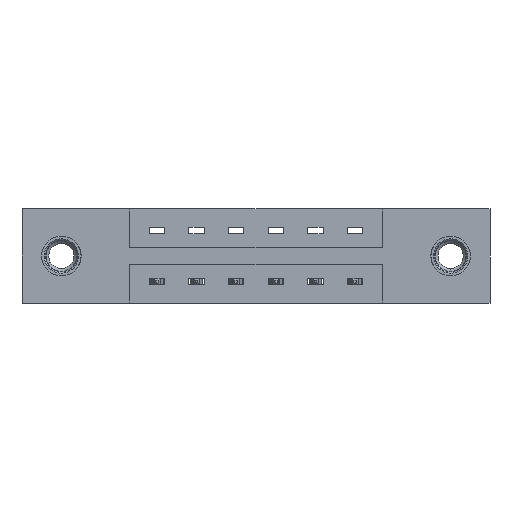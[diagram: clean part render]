
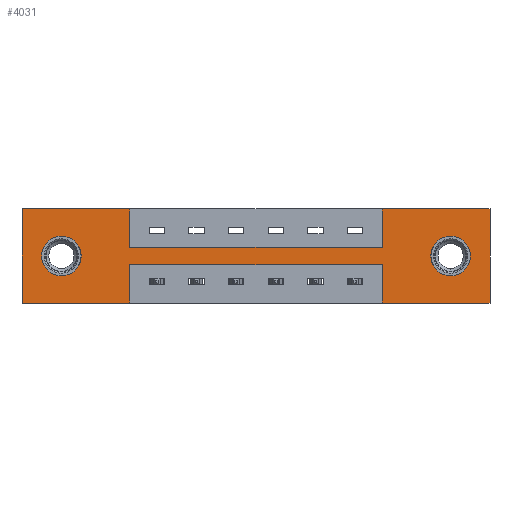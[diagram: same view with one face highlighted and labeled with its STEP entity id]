
A CAD part, front view. The second image highlights one B-rep face of the part: STEP entity #4031.
In plain terms, the highlighted planar face has unit normal (0, -1, 0).
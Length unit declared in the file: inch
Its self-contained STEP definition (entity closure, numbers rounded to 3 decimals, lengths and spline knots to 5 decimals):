
#107 = VECTOR ( 'NONE', #5665, 39.37008 ) ;
#125 = CARTESIAN_POINT ( 'NONE',  ( 0.425, 0., 0. ) ) ;
#155 = CARTESIAN_POINT ( 'NONE',  ( 1.842, 0., 0. ) ) ;
#157 = VERTEX_POINT ( 'NONE', #7164 ) ;
#264 = LINE ( 'NONE', #3424, #6249 ) ;
#421 = FACE_OUTER_BOUND ( 'NONE', #9651, .T. ) ;
#451 = DIRECTION ( 'NONE',  ( 0., 0., 1. ) ) ;
#482 = VERTEX_POINT ( 'NONE', #5175 ) ;
#483 = ORIENTED_EDGE ( 'NONE', *, *, #7003, .T. ) ;
#486 = LINE ( 'NONE', #1958, #2601 ) ;
#682 = VECTOR ( 'NONE', #8578, 39.37008 ) ;
#704 = LINE ( 'NONE', #2115, #1586 ) ;
#732 = DIRECTION ( 'NONE',  ( 0., 0., -1. ) ) ;
#839 = LINE ( 'NONE', #4768, #1840 ) ;
#875 = EDGE_CURVE ( 'NONE', #3739, #8464, #264, .T. ) ;
#1070 = VECTOR ( 'NONE', #9857, 39.37008 ) ;
#1173 = ORIENTED_EDGE ( 'NONE', *, *, #875, .F. ) ;
#1215 = VERTEX_POINT ( 'NONE', #9106 ) ;
#1236 = AXIS2_PLACEMENT_3D ( 'NONE', #1918, #8223, #9912 ) ;
#1338 = CARTESIAN_POINT ( 'NONE',  ( 0.425, 0., -0.37 ) ) ;
#1411 = EDGE_LOOP ( 'NONE', ( #483, #3594 ) ) ;
#1547 = EDGE_CURVE ( 'NONE', #9848, #2451, #4729, .T. ) ;
#1586 = VECTOR ( 'NONE', #451, 39.37008 ) ;
#1597 = DIRECTION ( 'NONE',  ( 0., 0., 1. ) ) ;
#1738 = VERTEX_POINT ( 'NONE', #2378 ) ;
#1745 = VERTEX_POINT ( 'NONE', #4076 ) ;
#1784 = DIRECTION ( 'NONE',  ( 0., 0., 1. ) ) ;
#1840 = VECTOR ( 'NONE', #1597, 39.37008 ) ;
#1918 = CARTESIAN_POINT ( 'NONE',  ( 1.687, 0., -0.185 ) ) ;
#1941 = DIRECTION ( 'NONE',  ( 0., -1., 0. ) ) ;
#1958 = CARTESIAN_POINT ( 'NONE',  ( 0., 0., -0.37 ) ) ;
#2009 = CARTESIAN_POINT ( 'NONE',  ( 0., 0., -0.37 ) ) ;
#2115 = CARTESIAN_POINT ( 'NONE',  ( 1.417, 0., 0. ) ) ;
#2192 = EDGE_CURVE ( 'NONE', #8464, #482, #3199, .T. ) ;
#2226 = DIRECTION ( 'NONE',  ( 1., 0., 0. ) ) ;
#2378 = CARTESIAN_POINT ( 'NONE',  ( 1.417, 0., -0.37 ) ) ;
#2384 = ORIENTED_EDGE ( 'NONE', *, *, #6631, .F. ) ;
#2394 = DIRECTION ( 'NONE',  ( 0., 1., 0. ) ) ;
#2451 = VERTEX_POINT ( 'NONE', #5269 ) ;
#2475 = EDGE_CURVE ( 'NONE', #482, #9816, #704, .T. ) ;
#2498 = CARTESIAN_POINT ( 'NONE',  ( 0.425, 0., -0.22 ) ) ;
#2515 = ORIENTED_EDGE ( 'NONE', *, *, #2475, .F. ) ;
#2528 = FACE_BOUND ( 'NONE', #1411, .T. ) ;
#2574 = CARTESIAN_POINT ( 'NONE',  ( 0., 0., 0. ) ) ;
#2601 = VECTOR ( 'NONE', #7566, 39.37008 ) ;
#2655 = CIRCLE ( 'NONE', #9099, 0.078 ) ;
#2710 = CIRCLE ( 'NONE', #3283, 0.078 ) ;
#2769 = LINE ( 'NONE', #2574, #5396 ) ;
#2834 = LINE ( 'NONE', #3782, #3086 ) ;
#2854 = LINE ( 'NONE', #5039, #9895 ) ;
#3024 = FACE_BOUND ( 'NONE', #3153, .T. ) ;
#3029 = CARTESIAN_POINT ( 'NONE',  ( 0.425, 0., -0.15 ) ) ;
#3086 = VECTOR ( 'NONE', #2226, 39.37008 ) ;
#3153 = EDGE_LOOP ( 'NONE', ( #8442, #5139 ) ) ;
#3199 = LINE ( 'NONE', #4795, #107 ) ;
#3210 = EDGE_CURVE ( 'NONE', #7838, #157, #9429, .T. ) ;
#3283 = AXIS2_PLACEMENT_3D ( 'NONE', #8961, #9764, #1784 ) ;
#3424 = CARTESIAN_POINT ( 'NONE',  ( 0.425, 0., 0. ) ) ;
#3465 = DIRECTION ( 'NONE',  ( 0., 0., -1. ) ) ;
#3594 = ORIENTED_EDGE ( 'NONE', *, *, #3713, .T. ) ;
#3713 = EDGE_CURVE ( 'NONE', #6350, #4746, #2655, .T. ) ;
#3739 = VERTEX_POINT ( 'NONE', #125 ) ;
#3782 = CARTESIAN_POINT ( 'NONE',  ( 0., 0., 0. ) ) ;
#3869 = VECTOR ( 'NONE', #6880, 39.37008 ) ;
#4019 = VECTOR ( 'NONE', #7086, 39.37008 ) ;
#4031 = ADVANCED_FACE ( 'NONE', ( #3024, #2528, #421 ), #8391, .T. ) ;
#4065 = DIRECTION ( 'NONE',  ( 1., 0., 0. ) ) ;
#4076 = CARTESIAN_POINT ( 'NONE',  ( 1.417, 0., -0.22 ) ) ;
#4135 = ORIENTED_EDGE ( 'NONE', *, *, #6311, .F. ) ;
#4234 = DIRECTION ( 'NONE',  ( 0., 0., -1. ) ) ;
#4255 = EDGE_CURVE ( 'NONE', #2451, #9848, #7679, .T. ) ;
#4355 = EDGE_CURVE ( 'NONE', #9816, #7743, #2769, .T. ) ;
#4473 = VERTEX_POINT ( 'NONE', #7274 ) ;
#4729 = CIRCLE ( 'NONE', #1236, 0.078 ) ;
#4732 = CARTESIAN_POINT ( 'NONE',  ( 0., 0., 0. ) ) ;
#4739 = AXIS2_PLACEMENT_3D ( 'NONE', #9506, #2394, #732 ) ;
#4746 = VERTEX_POINT ( 'NONE', #6963 ) ;
#4768 = CARTESIAN_POINT ( 'NONE',  ( 1.417, 0., -0.37 ) ) ;
#4795 = CARTESIAN_POINT ( 'NONE',  ( 0.425, 0., -0.15 ) ) ;
#4933 = CARTESIAN_POINT ( 'NONE',  ( 1.687, 0., -0.263 ) ) ;
#5039 = CARTESIAN_POINT ( 'NONE',  ( 1.842, 0., 0. ) ) ;
#5139 = ORIENTED_EDGE ( 'NONE', *, *, #1547, .T. ) ;
#5154 = EDGE_CURVE ( 'NONE', #4473, #1738, #8388, .T. ) ;
#5175 = CARTESIAN_POINT ( 'NONE',  ( 1.417, 0., -0.15 ) ) ;
#5269 = CARTESIAN_POINT ( 'NONE',  ( 1.687, 0., -0.107 ) ) ;
#5276 = CARTESIAN_POINT ( 'NONE',  ( 0., 0., -0.37 ) ) ;
#5392 = ORIENTED_EDGE ( 'NONE', *, *, #5154, .F. ) ;
#5396 = VECTOR ( 'NONE', #4065, 39.37008 ) ;
#5573 = DIRECTION ( 'NONE',  ( 0., 0., 1. ) ) ;
#5665 = DIRECTION ( 'NONE',  ( 1., 0., 0. ) ) ;
#5760 = CARTESIAN_POINT ( 'NONE',  ( 1.417, 0., 0. ) ) ;
#6031 = EDGE_CURVE ( 'NONE', #8325, #1215, #8273, .T. ) ;
#6127 = CARTESIAN_POINT ( 'NONE',  ( 0., 0., -0.37 ) ) ;
#6249 = VECTOR ( 'NONE', #4234, 39.37008 ) ;
#6311 = EDGE_CURVE ( 'NONE', #7743, #4473, #2854, .T. ) ;
#6350 = VERTEX_POINT ( 'NONE', #6685 ) ;
#6411 = DIRECTION ( 'NONE',  ( 0., 1., 0. ) ) ;
#6590 = LINE ( 'NONE', #7442, #1070 ) ;
#6631 = EDGE_CURVE ( 'NONE', #157, #8325, #486, .T. ) ;
#6685 = CARTESIAN_POINT ( 'NONE',  ( 0.155, 0., -0.263 ) ) ;
#6880 = DIRECTION ( 'NONE',  ( -1., 0., 0. ) ) ;
#6963 = CARTESIAN_POINT ( 'NONE',  ( 0.155, 0., -0.107 ) ) ;
#7003 = EDGE_CURVE ( 'NONE', #4746, #6350, #2710, .T. ) ;
#7062 = ORIENTED_EDGE ( 'NONE', *, *, #3210, .F. ) ;
#7086 = DIRECTION ( 'NONE',  ( 0., 0., 1. ) ) ;
#7164 = CARTESIAN_POINT ( 'NONE',  ( 0.425, 0., -0.37 ) ) ;
#7246 = ORIENTED_EDGE ( 'NONE', *, *, #4355, .F. ) ;
#7274 = CARTESIAN_POINT ( 'NONE',  ( 1.842, 0., -0.37 ) ) ;
#7296 = AXIS2_PLACEMENT_3D ( 'NONE', #2009, #1941, #8351 ) ;
#7442 = CARTESIAN_POINT ( 'NONE',  ( 0.425, 0., -0.22 ) ) ;
#7566 = DIRECTION ( 'NONE',  ( -1., 0., 0. ) ) ;
#7661 = EDGE_CURVE ( 'NONE', #1215, #3739, #2834, .T. ) ;
#7679 = CIRCLE ( 'NONE', #4739, 0.078 ) ;
#7743 = VERTEX_POINT ( 'NONE', #155 ) ;
#7826 = ORIENTED_EDGE ( 'NONE', *, *, #7661, .F. ) ;
#7838 = VERTEX_POINT ( 'NONE', #2498 ) ;
#8040 = CARTESIAN_POINT ( 'NONE',  ( 0.155, 0., -0.185 ) ) ;
#8104 = ORIENTED_EDGE ( 'NONE', *, *, #6031, .F. ) ;
#8138 = EDGE_CURVE ( 'NONE', #1738, #1745, #839, .T. ) ;
#8223 = DIRECTION ( 'NONE',  ( 0., 1., 0. ) ) ;
#8273 = LINE ( 'NONE', #4732, #4019 ) ;
#8325 = VERTEX_POINT ( 'NONE', #6127 ) ;
#8351 = DIRECTION ( 'NONE',  ( 0., 0., -1. ) ) ;
#8388 = LINE ( 'NONE', #5276, #3869 ) ;
#8391 = PLANE ( 'NONE',  #7296 ) ;
#8442 = ORIENTED_EDGE ( 'NONE', *, *, #4255, .T. ) ;
#8464 = VERTEX_POINT ( 'NONE', #3029 ) ;
#8578 = DIRECTION ( 'NONE',  ( 0., 0., -1. ) ) ;
#8683 = ORIENTED_EDGE ( 'NONE', *, *, #9445, .F. ) ;
#8961 = CARTESIAN_POINT ( 'NONE',  ( 0.155, 0., -0.185 ) ) ;
#9099 = AXIS2_PLACEMENT_3D ( 'NONE', #8040, #6411, #5573 ) ;
#9106 = CARTESIAN_POINT ( 'NONE',  ( 0., 0., 0. ) ) ;
#9429 = LINE ( 'NONE', #1338, #682 ) ;
#9445 = EDGE_CURVE ( 'NONE', #1745, #7838, #6590, .T. ) ;
#9506 = CARTESIAN_POINT ( 'NONE',  ( 1.687, 0., -0.185 ) ) ;
#9651 = EDGE_LOOP ( 'NONE', ( #7062, #8683, #10034, #5392, #4135, #7246, #2515, #10084, #1173, #7826, #8104, #2384 ) ) ;
#9764 = DIRECTION ( 'NONE',  ( 0., 1., 0. ) ) ;
#9816 = VERTEX_POINT ( 'NONE', #5760 ) ;
#9848 = VERTEX_POINT ( 'NONE', #4933 ) ;
#9857 = DIRECTION ( 'NONE',  ( -1., 0., 0. ) ) ;
#9895 = VECTOR ( 'NONE', #3465, 39.37008 ) ;
#9912 = DIRECTION ( 'NONE',  ( 0., 0., -1. ) ) ;
#10034 = ORIENTED_EDGE ( 'NONE', *, *, #8138, .F. ) ;
#10084 = ORIENTED_EDGE ( 'NONE', *, *, #2192, .F. ) ;
